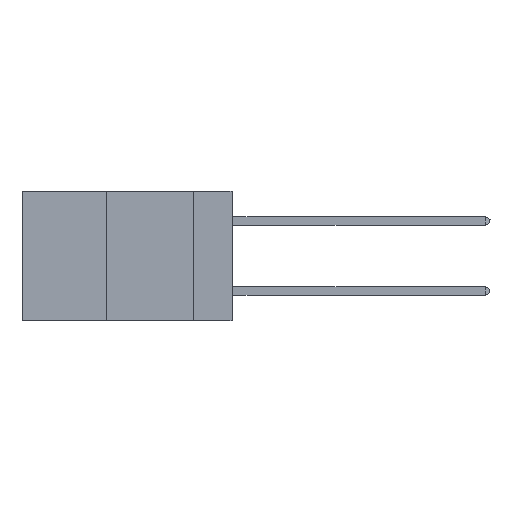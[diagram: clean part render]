
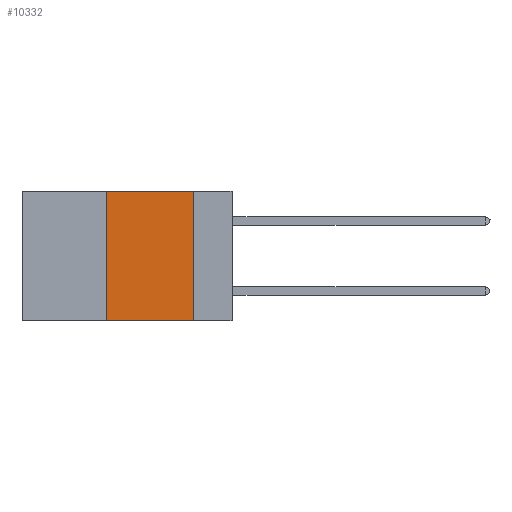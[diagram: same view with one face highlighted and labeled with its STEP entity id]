
A CAD part, left-side view. The second image highlights one B-rep face of the part: STEP entity #10332.
In plain terms, the highlighted planar face has unit normal (-1, 0, 0).
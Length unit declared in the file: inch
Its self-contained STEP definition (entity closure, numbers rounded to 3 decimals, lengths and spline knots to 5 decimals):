
#106 = ORIENTED_EDGE ( 'NONE', *, *, #17258, .F. ) ;
#1925 = LINE ( 'NONE', #15959, #6276 ) ;
#2158 = CARTESIAN_POINT ( 'NONE',  ( 0., 0.36, 0. ) ) ;
#2331 = VERTEX_POINT ( 'NONE', #11173 ) ;
#2409 = AXIS2_PLACEMENT_3D ( 'NONE', #8257, #19892, #17646 ) ;
#2417 = CARTESIAN_POINT ( 'NONE',  ( 0., 0.11, -0.37 ) ) ;
#4210 = PLANE ( 'NONE',  #2409 ) ;
#5683 = DIRECTION ( 'NONE',  ( 0., 0., -1. ) ) ;
#6276 = VECTOR ( 'NONE', #25028, 39.37008 ) ;
#8257 = CARTESIAN_POINT ( 'NONE',  ( 0., 0.6, 0. ) ) ;
#9270 = CARTESIAN_POINT ( 'NONE',  ( 0., 0.36, 0. ) ) ;
#10332 = ADVANCED_FACE ( 'NONE', ( #15287 ), #4210, .F. ) ;
#10394 = VERTEX_POINT ( 'NONE', #2417 ) ;
#10582 = EDGE_LOOP ( 'NONE', ( #20977, #28335, #106, #18021 ) ) ;
#11173 = CARTESIAN_POINT ( 'NONE',  ( 0., 0.11, 0. ) ) ;
#12104 = CARTESIAN_POINT ( 'NONE',  ( 0., 0.11, 0. ) ) ;
#15287 = FACE_OUTER_BOUND ( 'NONE', #10582, .T. ) ;
#15959 = CARTESIAN_POINT ( 'NONE',  ( 0., 0.6, -0.37 ) ) ;
#16333 = VECTOR ( 'NONE', #5683, 39.37008 ) ;
#17258 = EDGE_CURVE ( 'NONE', #22627, #24954, #27452, .T. ) ;
#17646 = DIRECTION ( 'NONE',  ( 0., 0., -1. ) ) ;
#18021 = ORIENTED_EDGE ( 'NONE', *, *, #20550, .T. ) ;
#18377 = DIRECTION ( 'NONE',  ( 0., 0., 1. ) ) ;
#19268 = LINE ( 'NONE', #26101, #20157 ) ;
#19892 = DIRECTION ( 'NONE',  ( 1., 0., 0. ) ) ;
#20157 = VECTOR ( 'NONE', #28341, 39.37008 ) ;
#20550 = EDGE_CURVE ( 'NONE', #22627, #10394, #1925, .T. ) ;
#20891 = LINE ( 'NONE', #12104, #16333 ) ;
#20905 = VECTOR ( 'NONE', #18377, 39.37008 ) ;
#20977 = ORIENTED_EDGE ( 'NONE', *, *, #21701, .F. ) ;
#21701 = EDGE_CURVE ( 'NONE', #2331, #10394, #20891, .T. ) ;
#21912 = CARTESIAN_POINT ( 'NONE',  ( 0., 0.36, -0.37 ) ) ;
#22360 = EDGE_CURVE ( 'NONE', #24954, #2331, #19268, .T. ) ;
#22627 = VERTEX_POINT ( 'NONE', #21912 ) ;
#24954 = VERTEX_POINT ( 'NONE', #2158 ) ;
#25028 = DIRECTION ( 'NONE',  ( 0., -1., 0. ) ) ;
#26101 = CARTESIAN_POINT ( 'NONE',  ( 0., 0.6, 0. ) ) ;
#27452 = LINE ( 'NONE', #9270, #20905 ) ;
#28335 = ORIENTED_EDGE ( 'NONE', *, *, #22360, .F. ) ;
#28341 = DIRECTION ( 'NONE',  ( 0., -1., 0. ) ) ;
